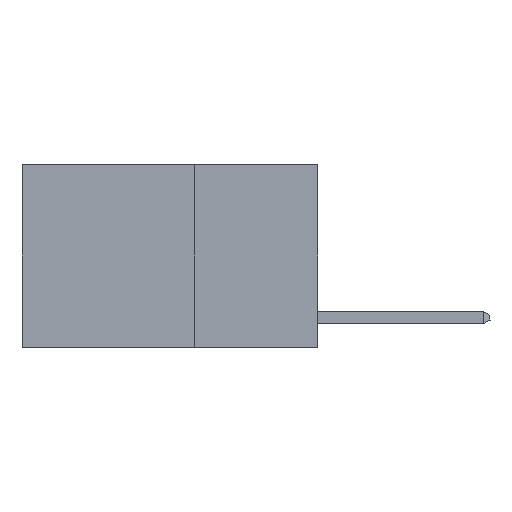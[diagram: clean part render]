
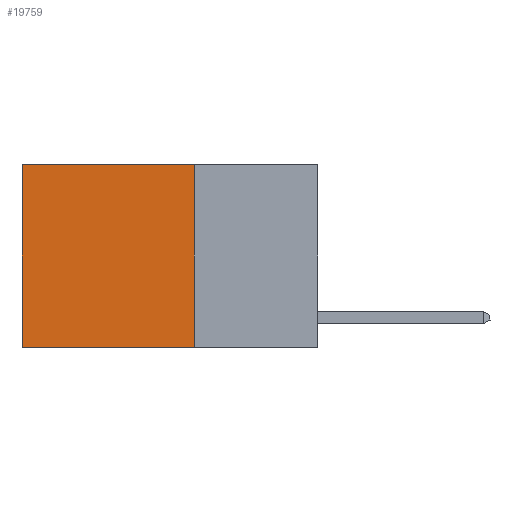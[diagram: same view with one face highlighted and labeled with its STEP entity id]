
A CAD part, left-side view. The second image highlights one B-rep face of the part: STEP entity #19759.
In plain terms, the highlighted planar face has unit normal (-1, 0, 0).
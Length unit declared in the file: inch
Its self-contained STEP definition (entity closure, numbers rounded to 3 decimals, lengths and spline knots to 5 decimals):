
#868 = CARTESIAN_POINT ( 'NONE',  ( 0.2625, 0.25, 0. ) ) ;
#1588 = CARTESIAN_POINT ( 'NONE',  ( 0.2625, 0.6, -0.37 ) ) ;
#2424 = VECTOR ( 'NONE', #4873, 39.37008 ) ;
#4208 = DIRECTION ( 'NONE',  ( 0., 0., -1. ) ) ;
#4779 = VECTOR ( 'NONE', #4208, 39.37008 ) ;
#4873 = DIRECTION ( 'NONE',  ( 0., 1., 0. ) ) ;
#5114 = EDGE_CURVE ( 'NONE', #22609, #20998, #21503, .T. ) ;
#5338 = ORIENTED_EDGE ( 'NONE', *, *, #19643, .F. ) ;
#7172 = DIRECTION ( 'NONE',  ( 0., 0., -1. ) ) ;
#7203 = LINE ( 'NONE', #16942, #2424 ) ;
#7269 = DIRECTION ( 'NONE',  ( 0., 1., 0. ) ) ;
#7336 = ORIENTED_EDGE ( 'NONE', *, *, #19792, .T. ) ;
#7963 = CARTESIAN_POINT ( 'NONE',  ( 0.2625, 0.6, 0. ) ) ;
#7994 = AXIS2_PLACEMENT_3D ( 'NONE', #21175, #19227, #7172 ) ;
#10469 = CARTESIAN_POINT ( 'NONE',  ( 0.2625, 0.6, 0. ) ) ;
#10561 = LINE ( 'NONE', #10469, #20632 ) ;
#10677 = FACE_OUTER_BOUND ( 'NONE', #13715, .T. ) ;
#12853 = VERTEX_POINT ( 'NONE', #7963 ) ;
#13715 = EDGE_LOOP ( 'NONE', ( #21425, #5338, #20728, #7336 ) ) ;
#15158 = PLANE ( 'NONE',  #7994 ) ;
#16249 = CARTESIAN_POINT ( 'NONE',  ( 0.2625, 0.25, 0. ) ) ;
#16942 = CARTESIAN_POINT ( 'NONE',  ( 0.2625, 0.25, -0.37 ) ) ;
#18144 = CARTESIAN_POINT ( 'NONE',  ( 0.2625, 0.25, -0.37 ) ) ;
#19227 = DIRECTION ( 'NONE',  ( 1., 0., 0. ) ) ;
#19482 = VECTOR ( 'NONE', #7269, 39.37008 ) ;
#19643 = EDGE_CURVE ( 'NONE', #20998, #22880, #7203, .T. ) ;
#19759 = ADVANCED_FACE ( 'NONE', ( #10677 ), #15158, .F. ) ;
#19792 = EDGE_CURVE ( 'NONE', #22609, #12853, #24830, .T. ) ;
#20632 = VECTOR ( 'NONE', #24538, 39.37008 ) ;
#20728 = ORIENTED_EDGE ( 'NONE', *, *, #5114, .F. ) ;
#20998 = VERTEX_POINT ( 'NONE', #18144 ) ;
#21175 = CARTESIAN_POINT ( 'NONE',  ( 0.2625, 0.25, 0. ) ) ;
#21267 = CARTESIAN_POINT ( 'NONE',  ( 0.2625, 0.25, 0. ) ) ;
#21425 = ORIENTED_EDGE ( 'NONE', *, *, #21738, .T. ) ;
#21503 = LINE ( 'NONE', #16249, #4779 ) ;
#21738 = EDGE_CURVE ( 'NONE', #12853, #22880, #10561, .T. ) ;
#22609 = VERTEX_POINT ( 'NONE', #868 ) ;
#22880 = VERTEX_POINT ( 'NONE', #1588 ) ;
#24538 = DIRECTION ( 'NONE',  ( 0., 0., -1. ) ) ;
#24830 = LINE ( 'NONE', #21267, #19482 ) ;
